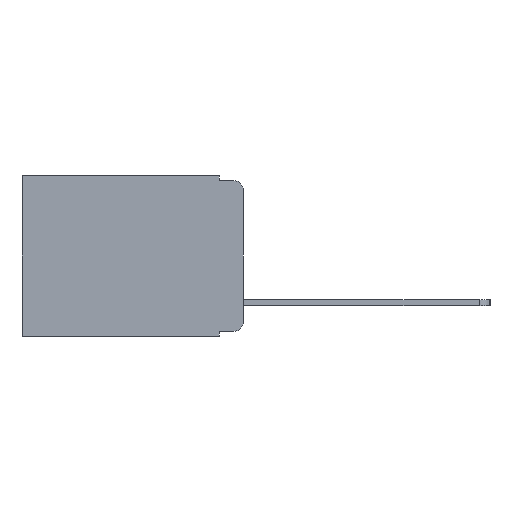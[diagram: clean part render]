
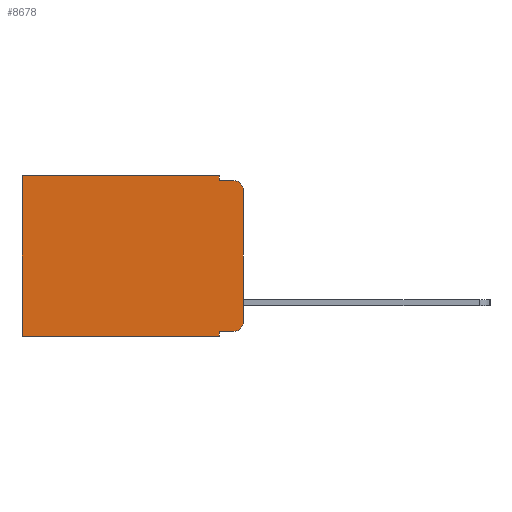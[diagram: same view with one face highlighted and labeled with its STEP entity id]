
A CAD part, left-side view. The second image highlights one B-rep face of the part: STEP entity #8678.
In plain terms, the highlighted planar face has unit normal (-1, 0, 0).
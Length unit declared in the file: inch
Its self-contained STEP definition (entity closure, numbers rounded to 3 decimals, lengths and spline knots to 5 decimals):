
#2 = CIRCLE ( 'NONE', #5040, 0.02 ) ;
#270 = CARTESIAN_POINT ( 'NONE',  ( 0.298, 0., 0. ) ) ;
#952 = DIRECTION ( 'NONE',  ( 0., -1., 0. ) ) ;
#1449 = LINE ( 'NONE', #4125, #5961 ) ;
#1475 = ORIENTED_EDGE ( 'NONE', *, *, #8891, .T. ) ;
#1717 = CIRCLE ( 'NONE', #8852, 0.02 ) ;
#2007 = CARTESIAN_POINT ( 'NONE',  ( 0.298, 0.02, -0.03 ) ) ;
#2213 = VECTOR ( 'NONE', #8316, 39.37008 ) ;
#2297 = ORIENTED_EDGE ( 'NONE', *, *, #8389, .F. ) ;
#2344 = LINE ( 'NONE', #3601, #10955 ) ;
#2411 = VERTEX_POINT ( 'NONE', #7264 ) ;
#2617 = DIRECTION ( 'NONE',  ( 0., 0., -1. ) ) ;
#2775 = VERTEX_POINT ( 'NONE', #3583 ) ;
#2955 = DIRECTION ( 'NONE',  ( 0., 0., -1. ) ) ;
#3040 = VERTEX_POINT ( 'NONE', #10874 ) ;
#3467 = VERTEX_POINT ( 'NONE', #6254 ) ;
#3583 = CARTESIAN_POINT ( 'NONE',  ( 0.298, 0.02, -0.01 ) ) ;
#3601 = CARTESIAN_POINT ( 'NONE',  ( 0.298, 0.051, 0. ) ) ;
#3762 = CARTESIAN_POINT ( 'NONE',  ( 0.298, 0.051, -0.343 ) ) ;
#3805 = CARTESIAN_POINT ( 'NONE',  ( 0.298, 0., -0.343 ) ) ;
#3936 = ORIENTED_EDGE ( 'NONE', *, *, #9904, .F. ) ;
#3996 = ORIENTED_EDGE ( 'NONE', *, *, #5667, .T. ) ;
#4125 = CARTESIAN_POINT ( 'NONE',  ( 0.298, 0.051, -0.01 ) ) ;
#4140 = VERTEX_POINT ( 'NONE', #8571 ) ;
#4346 = VERTEX_POINT ( 'NONE', #6462 ) ;
#4414 = EDGE_CURVE ( 'NONE', #3040, #5057, #10346, .T. ) ;
#4438 = AXIS2_PLACEMENT_3D ( 'NONE', #5399, #10979, #6220 ) ;
#4829 = CARTESIAN_POINT ( 'NONE',  ( 0.298, 0., 0. ) ) ;
#4952 = LINE ( 'NONE', #8382, #2213 ) ;
#4964 = VECTOR ( 'NONE', #9595, 39.37008 ) ;
#4987 = DIRECTION ( 'NONE',  ( 0., 1., 0. ) ) ;
#5040 = AXIS2_PLACEMENT_3D ( 'NONE', #10633, #10296, #9325 ) ;
#5057 = VERTEX_POINT ( 'NONE', #10677 ) ;
#5367 = VECTOR ( 'NONE', #952, 39.37008 ) ;
#5399 = CARTESIAN_POINT ( 'NONE',  ( 0.298, 0., 0. ) ) ;
#5400 = ORIENTED_EDGE ( 'NONE', *, *, #7281, .T. ) ;
#5588 = FACE_OUTER_BOUND ( 'NONE', #5943, .T. ) ;
#5635 = LINE ( 'NONE', #9794, #5367 ) ;
#5667 = EDGE_CURVE ( 'NONE', #3467, #6313, #2, .T. ) ;
#5943 = EDGE_LOOP ( 'NONE', ( #3936, #1475, #2297, #9871, #8922, #5400, #9368, #6292, #10773, #3996 ) ) ;
#5961 = VECTOR ( 'NONE', #10716, 39.37008 ) ;
#6204 = EDGE_CURVE ( 'NONE', #7920, #3467, #5635, .T. ) ;
#6220 = DIRECTION ( 'NONE',  ( 0., 0., -1. ) ) ;
#6232 = CARTESIAN_POINT ( 'NONE',  ( 0.298, 0.051, -0.333 ) ) ;
#6254 = CARTESIAN_POINT ( 'NONE',  ( 0.298, 0.02, -0.333 ) ) ;
#6292 = ORIENTED_EDGE ( 'NONE', *, *, #6727, .F. ) ;
#6313 = VERTEX_POINT ( 'NONE', #9736 ) ;
#6321 = LINE ( 'NONE', #3805, #10026 ) ;
#6462 = CARTESIAN_POINT ( 'NONE',  ( 0.298, 0.051, -0.01 ) ) ;
#6727 = EDGE_CURVE ( 'NONE', #7920, #9668, #9004, .T. ) ;
#7264 = CARTESIAN_POINT ( 'NONE',  ( 0.298, 0.473, -0.343 ) ) ;
#7281 = EDGE_CURVE ( 'NONE', #5057, #2411, #4952, .T. ) ;
#7325 = LINE ( 'NONE', #270, #7572 ) ;
#7402 = DIRECTION ( 'NONE',  ( 0., 0., -1. ) ) ;
#7572 = VECTOR ( 'NONE', #7402, 39.37008 ) ;
#7821 = EDGE_CURVE ( 'NONE', #3040, #4346, #2344, .T. ) ;
#7920 = VERTEX_POINT ( 'NONE', #6232 ) ;
#8056 = DIRECTION ( 'NONE',  ( -1., 0., 0. ) ) ;
#8274 = VECTOR ( 'NONE', #4987, 39.37008 ) ;
#8316 = DIRECTION ( 'NONE',  ( 0., 0., -1. ) ) ;
#8382 = CARTESIAN_POINT ( 'NONE',  ( 0.298, 0.473, 0. ) ) ;
#8389 = EDGE_CURVE ( 'NONE', #4346, #2775, #1449, .T. ) ;
#8571 = CARTESIAN_POINT ( 'NONE',  ( 0.298, 0., -0.03 ) ) ;
#8626 = PLANE ( 'NONE',  #4438 ) ;
#8678 = ADVANCED_FACE ( 'NONE', ( #5588 ), #8626, .F. ) ;
#8813 = DIRECTION ( 'NONE',  ( 0., 1., 0. ) ) ;
#8852 = AXIS2_PLACEMENT_3D ( 'NONE', #2007, #8056, #2955 ) ;
#8891 = EDGE_CURVE ( 'NONE', #4140, #2775, #1717, .T. ) ;
#8922 = ORIENTED_EDGE ( 'NONE', *, *, #4414, .T. ) ;
#9004 = LINE ( 'NONE', #9297, #4964 ) ;
#9297 = CARTESIAN_POINT ( 'NONE',  ( 0.298, 0.051, 0. ) ) ;
#9325 = DIRECTION ( 'NONE',  ( 0., 0., -1. ) ) ;
#9368 = ORIENTED_EDGE ( 'NONE', *, *, #9703, .F. ) ;
#9595 = DIRECTION ( 'NONE',  ( 0., 0., -1. ) ) ;
#9668 = VERTEX_POINT ( 'NONE', #3762 ) ;
#9703 = EDGE_CURVE ( 'NONE', #9668, #2411, #6321, .T. ) ;
#9736 = CARTESIAN_POINT ( 'NONE',  ( 0.298, 0., -0.313 ) ) ;
#9794 = CARTESIAN_POINT ( 'NONE',  ( 0.298, 0.051, -0.333 ) ) ;
#9871 = ORIENTED_EDGE ( 'NONE', *, *, #7821, .F. ) ;
#9904 = EDGE_CURVE ( 'NONE', #4140, #6313, #7325, .T. ) ;
#10026 = VECTOR ( 'NONE', #8813, 39.37008 ) ;
#10296 = DIRECTION ( 'NONE',  ( -1., 0., 0. ) ) ;
#10346 = LINE ( 'NONE', #4829, #8274 ) ;
#10633 = CARTESIAN_POINT ( 'NONE',  ( 0.298, 0.02, -0.313 ) ) ;
#10677 = CARTESIAN_POINT ( 'NONE',  ( 0.298, 0.473, 0. ) ) ;
#10716 = DIRECTION ( 'NONE',  ( 0., -1., 0. ) ) ;
#10773 = ORIENTED_EDGE ( 'NONE', *, *, #6204, .T. ) ;
#10874 = CARTESIAN_POINT ( 'NONE',  ( 0.298, 0.051, 0. ) ) ;
#10955 = VECTOR ( 'NONE', #2617, 39.37008 ) ;
#10979 = DIRECTION ( 'NONE',  ( 1., 0., 0. ) ) ;
